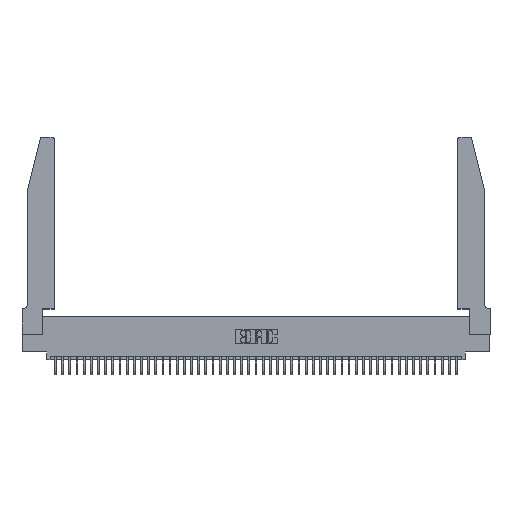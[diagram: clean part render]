
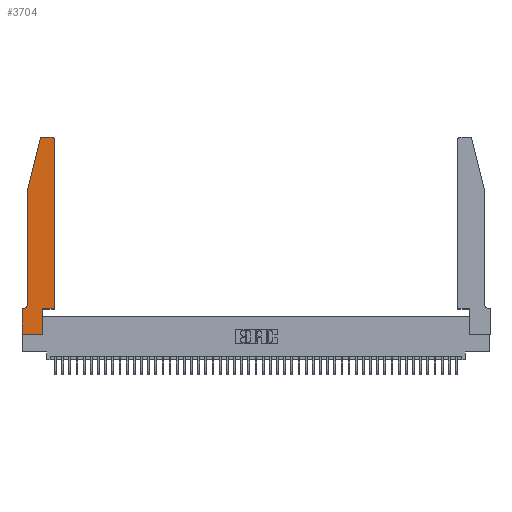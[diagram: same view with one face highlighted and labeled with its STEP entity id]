
A CAD part, top view. The second image highlights one B-rep face of the part: STEP entity #3704.
In plain terms, the highlighted planar face has unit normal (0, 0, 1).
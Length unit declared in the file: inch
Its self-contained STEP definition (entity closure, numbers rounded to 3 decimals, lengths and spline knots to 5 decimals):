
#149 = DIRECTION ( 'NONE',  ( 0., 0., -1. ) ) ;
#652 = DIRECTION ( 'NONE',  ( -1., 0., 0. ) ) ;
#840 = CIRCLE ( 'NONE', #16907, 0.03 ) ;
#937 = CARTESIAN_POINT ( 'NONE',  ( 0.4505, 0.35, 0.37 ) ) ;
#1036 = VERTEX_POINT ( 'NONE', #3794 ) ;
#1077 = CARTESIAN_POINT ( 'NONE',  ( 0.4505, 0.35, 0.37 ) ) ;
#1171 = VERTEX_POINT ( 'NONE', #23718 ) ;
#1474 = CARTESIAN_POINT ( 'NONE',  ( 0.0755, 2., 0.37 ) ) ;
#1688 = VERTEX_POINT ( 'NONE', #28092 ) ;
#1716 = CARTESIAN_POINT ( 'NONE',  ( 0., 0., 0.37 ) ) ;
#1923 = ORIENTED_EDGE ( 'NONE', *, *, #15268, .T. ) ;
#2123 = ORIENTED_EDGE ( 'NONE', *, *, #20520, .T. ) ;
#2543 = VERTEX_POINT ( 'NONE', #4289 ) ;
#2964 = CARTESIAN_POINT ( 'NONE',  ( 0.4505, 0.35, 0.37 ) ) ;
#3191 = CARTESIAN_POINT ( 'NONE',  ( 0.0055, 0.35, 0.37 ) ) ;
#3704 = ADVANCED_FACE ( 'NONE', ( #40516 ), #40505, .T. ) ;
#3794 = CARTESIAN_POINT ( 'NONE',  ( 0., 0.35, 0.37 ) ) ;
#3983 = DIRECTION ( 'NONE',  ( -1., 0., 0. ) ) ;
#4022 = CARTESIAN_POINT ( 'NONE',  ( 0., 0., 0.37 ) ) ;
#4117 = EDGE_CURVE ( 'NONE', #1036, #18458, #26180, .T. ) ;
#4141 = CARTESIAN_POINT ( 'NONE',  ( 0.284, 2.72, 0.37 ) ) ;
#4289 = CARTESIAN_POINT ( 'NONE',  ( 0.0755, 0.42, 0.37 ) ) ;
#4526 = CARTESIAN_POINT ( 'NONE',  ( 0.2865, 0., 0.37 ) ) ;
#5372 = VECTOR ( 'NONE', #13218, 39.37008 ) ;
#5481 = AXIS2_PLACEMENT_3D ( 'NONE', #10910, #21522, #25527 ) ;
#6067 = ORIENTED_EDGE ( 'NONE', *, *, #32051, .T. ) ;
#7522 = CARTESIAN_POINT ( 'NONE',  ( 0., 0., 0.37 ) ) ;
#8919 = CARTESIAN_POINT ( 'NONE',  ( 0.0755, 2., 0.37 ) ) ;
#9047 = EDGE_CURVE ( 'NONE', #38650, #16866, #39503, .T. ) ;
#10105 = LINE ( 'NONE', #4022, #12484 ) ;
#10519 = CARTESIAN_POINT ( 'NONE',  ( 0.2865, 0.35, 0.37 ) ) ;
#10910 = CARTESIAN_POINT ( 'NONE',  ( 0., 0.35, 0.37 ) ) ;
#11930 = ORIENTED_EDGE ( 'NONE', *, *, #19928, .T. ) ;
#12484 = VECTOR ( 'NONE', #45474, 39.37008 ) ;
#12603 = LINE ( 'NONE', #37420, #23885 ) ;
#12749 = VECTOR ( 'NONE', #20211, 39.37008 ) ;
#13218 = DIRECTION ( 'NONE',  ( 0., -1., 0. ) ) ;
#14672 = DIRECTION ( 'NONE',  ( -1., 0., 0. ) ) ;
#15268 = EDGE_CURVE ( 'NONE', #1688, #34757, #36761, .T. ) ;
#15477 = DIRECTION ( 'NONE',  ( 0., 0., 1. ) ) ;
#15873 = VERTEX_POINT ( 'NONE', #3191 ) ;
#16168 = LINE ( 'NONE', #2964, #45934 ) ;
#16866 = VERTEX_POINT ( 'NONE', #937 ) ;
#16907 = AXIS2_PLACEMENT_3D ( 'NONE', #19358, #30818, #19510 ) ;
#17030 = VERTEX_POINT ( 'NONE', #18082 ) ;
#17446 = ORIENTED_EDGE ( 'NONE', *, *, #18624, .T. ) ;
#17806 = VECTOR ( 'NONE', #3983, 39.37008 ) ;
#18082 = CARTESIAN_POINT ( 'NONE',  ( 0.4205, 2.75, 0.37 ) ) ;
#18458 = VERTEX_POINT ( 'NONE', #7522 ) ;
#18624 = EDGE_CURVE ( 'NONE', #1171, #1688, #33415, .T. ) ;
#19358 = CARTESIAN_POINT ( 'NONE',  ( 0.4205, 2.72, 0.37 ) ) ;
#19510 = DIRECTION ( 'NONE',  ( 1., 0., 0. ) ) ;
#19928 = EDGE_CURVE ( 'NONE', #18458, #27882, #10105, .T. ) ;
#20211 = DIRECTION ( 'NONE',  ( 1., 0., 0. ) ) ;
#20432 = LINE ( 'NONE', #42574, #39479 ) ;
#20518 = ORIENTED_EDGE ( 'NONE', *, *, #41507, .T. ) ;
#20520 = EDGE_CURVE ( 'NONE', #15873, #1036, #33230, .T. ) ;
#21522 = DIRECTION ( 'NONE',  ( 0., 0., 1. ) ) ;
#21743 = DIRECTION ( 'NONE',  ( 0., 1., 0. ) ) ;
#22251 = DIRECTION ( 'NONE',  ( 0., 1., 0. ) ) ;
#23718 = CARTESIAN_POINT ( 'NONE',  ( 0.284, 2.75, 0.37 ) ) ;
#23885 = VECTOR ( 'NONE', #22251, 39.37008 ) ;
#25052 = ORIENTED_EDGE ( 'NONE', *, *, #28362, .T. ) ;
#25527 = DIRECTION ( 'NONE',  ( 1., 0., 0. ) ) ;
#26004 = CARTESIAN_POINT ( 'NONE',  ( 0.4505, 2.72, 0.37 ) ) ;
#26180 = LINE ( 'NONE', #1716, #5372 ) ;
#27882 = VERTEX_POINT ( 'NONE', #4526 ) ;
#28092 = CARTESIAN_POINT ( 'NONE',  ( 0.25487, 2.72718, 0.37 ) ) ;
#28362 = EDGE_CURVE ( 'NONE', #2543, #15873, #44105, .T. ) ;
#29078 = ORIENTED_EDGE ( 'NONE', *, *, #45156, .T. ) ;
#30818 = DIRECTION ( 'NONE',  ( 0., 0., 1. ) ) ;
#31988 = ORIENTED_EDGE ( 'NONE', *, *, #37535, .T. ) ;
#32051 = EDGE_CURVE ( 'NONE', #17030, #1171, #20432, .T. ) ;
#33230 = LINE ( 'NONE', #46089, #17806 ) ;
#33415 = CIRCLE ( 'NONE', #38889, 0.03 ) ;
#33861 = VECTOR ( 'NONE', #39305, 39.37008 ) ;
#34730 = DIRECTION ( 'NONE',  ( 1., 0., 0. ) ) ;
#34757 = VERTEX_POINT ( 'NONE', #1474 ) ;
#35580 = VECTOR ( 'NONE', #37830, 39.37008 ) ;
#35980 = ORIENTED_EDGE ( 'NONE', *, *, #46692, .T. ) ;
#36761 = LINE ( 'NONE', #37511, #35580 ) ;
#37420 = CARTESIAN_POINT ( 'NONE',  ( 0.2865, 0.35, 0.37 ) ) ;
#37511 = CARTESIAN_POINT ( 'NONE',  ( 0.0755, 2., 0.37 ) ) ;
#37535 = EDGE_CURVE ( 'NONE', #16866, #42386, #16168, .T. ) ;
#37573 = CARTESIAN_POINT ( 'NONE',  ( 0.0055, 0.42, 0.37 ) ) ;
#37830 = DIRECTION ( 'NONE',  ( -0.239, -0.971, 0. ) ) ;
#38650 = VERTEX_POINT ( 'NONE', #10519 ) ;
#38889 = AXIS2_PLACEMENT_3D ( 'NONE', #4141, #15477, #34730 ) ;
#39305 = DIRECTION ( 'NONE',  ( 0., -1., 0. ) ) ;
#39479 = VECTOR ( 'NONE', #652, 39.37008 ) ;
#39503 = LINE ( 'NONE', #1077, #12749 ) ;
#40399 = LINE ( 'NONE', #8919, #33861 ) ;
#40505 = PLANE ( 'NONE',  #5481 ) ;
#40516 = FACE_OUTER_BOUND ( 'NONE', #41543, .T. ) ;
#41507 = EDGE_CURVE ( 'NONE', #34757, #2543, #40399, .T. ) ;
#41543 = EDGE_LOOP ( 'NONE', ( #6067, #17446, #1923, #20518, #25052, #2123, #43528, #11930, #35980, #46220, #31988, #29078 ) ) ;
#42008 = AXIS2_PLACEMENT_3D ( 'NONE', #37573, #149, #14672 ) ;
#42386 = VERTEX_POINT ( 'NONE', #26004 ) ;
#42574 = CARTESIAN_POINT ( 'NONE',  ( 0.2605, 2.75, 0.37 ) ) ;
#43528 = ORIENTED_EDGE ( 'NONE', *, *, #4117, .T. ) ;
#44105 = CIRCLE ( 'NONE', #42008, 0.07 ) ;
#45156 = EDGE_CURVE ( 'NONE', #42386, #17030, #840, .T. ) ;
#45474 = DIRECTION ( 'NONE',  ( 1., 0., 0. ) ) ;
#45934 = VECTOR ( 'NONE', #21743, 39.37008 ) ;
#46089 = CARTESIAN_POINT ( 'NONE',  ( 0.0755, 0.35, 0.37 ) ) ;
#46220 = ORIENTED_EDGE ( 'NONE', *, *, #9047, .T. ) ;
#46692 = EDGE_CURVE ( 'NONE', #27882, #38650, #12603, .T. ) ;
